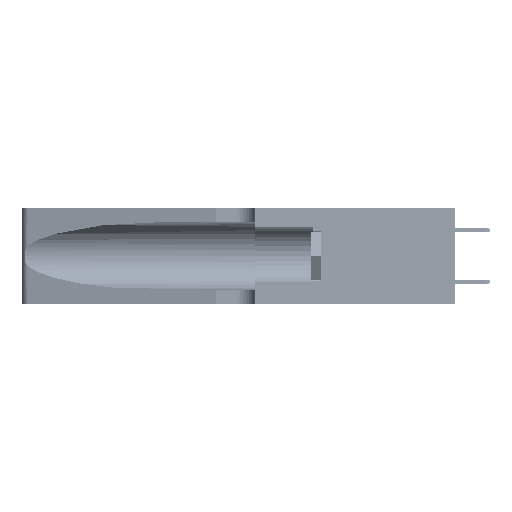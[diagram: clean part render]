
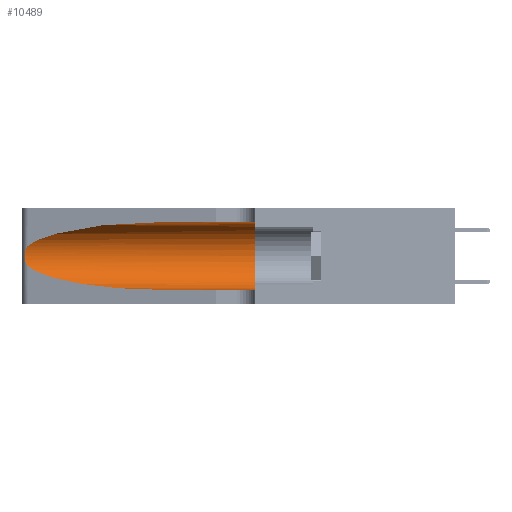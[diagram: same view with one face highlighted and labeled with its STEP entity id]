
A CAD part, left-side view. The second image highlights one B-rep face of the part: STEP entity #10489.
In plain terms, the highlighted cylindrical face has radius 3.308 mm (diameter 6.617 mm), a partial arc.
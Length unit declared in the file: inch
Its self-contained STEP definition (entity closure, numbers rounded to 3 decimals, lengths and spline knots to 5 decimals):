
#362 = ORIENTED_EDGE ( 'NONE', *, *, #37674, .F. ) ;
#454 = AXIS2_PLACEMENT_3D ( 'NONE', #43914, #44186, #11364 ) ;
#1135 = CARTESIAN_POINT ( 'NONE',  ( 0.1305, 1.61858, 0.05475 ) ) ;
#1635 = ORIENTED_EDGE ( 'NONE', *, *, #9774, .T. ) ;
#2029 = EDGE_CURVE ( 'NONE', #44877, #31511, #16882, .T. ) ;
#2065 = CARTESIAN_POINT ( 'NONE',  ( 0.1305, 0.35, 0.05475 ) ) ;
#3035 = DIRECTION ( 'NONE',  ( 0., -1., 0. ) ) ;
#4154 = CARTESIAN_POINT ( 'NONE',  ( 0.25555, 1.22994, 0.2215 ) ) ;
#4915 = VERTEX_POINT ( 'NONE', #21730 ) ;
#5447 =( BOUNDED_CURVE ( )  B_SPLINE_CURVE ( 3, ( #11576, #44661, #23521, #12105 ),
 .UNSPECIFIED., .F., .F. ) 
 B_SPLINE_CURVE_WITH_KNOTS ( ( 4, 4 ),
 ( 3.44316, 4.71239 ),
 .UNSPECIFIED. ) 
 CURVE ( )  GEOMETRIC_REPRESENTATION_ITEM ( )  RATIONAL_B_SPLINE_CURVE ( ( 1., 0.87, 0.87, 1. ) ) 
 REPRESENTATION_ITEM ( '' )  );
#7596 = CARTESIAN_POINT ( 'NONE',  ( 0.1305, 0.35, 0.31525 ) ) ;
#9774 = EDGE_CURVE ( 'NONE', #36606, #4915, #38628, .T. ) ;
#10489 = ADVANCED_FACE ( 'NONE', ( #14635 ), #14356, .F. ) ;
#10690 = CARTESIAN_POINT ( 'NONE',  ( 0.25487, 1.22718, 0.22369 ) ) ;
#10956 = CARTESIAN_POINT ( 'NONE',  ( 0.1305, 0.72297, 0.31525 ) ) ;
#11364 = DIRECTION ( 'NONE',  ( 0., 0., -1. ) ) ;
#11576 = CARTESIAN_POINT ( 'NONE',  ( 0.25487, 1.22718, 0.14631 ) ) ;
#11835 = ORIENTED_EDGE ( 'NONE', *, *, #2029, .T. ) ;
#12105 = CARTESIAN_POINT ( 'NONE',  ( 0.1305, 0.72297, 0.05475 ) ) ;
#12561 = CARTESIAN_POINT ( 'NONE',  ( 0.25487, 1.22718, 0.22369 ) ) ;
#12828 = CARTESIAN_POINT ( 'NONE',  ( 0.26075, 1.23896, 0.178 ) ) ;
#13082 = CARTESIAN_POINT ( 'NONE',  ( 0.26017, 1.23833, 0.17102 ) ) ;
#13103 = EDGE_CURVE ( 'NONE', #33153, #36606, #24790, .T. ) ;
#14356 = CYLINDRICAL_SURFACE ( 'NONE', #454, 0.13025 ) ;
#14635 = FACE_OUTER_BOUND ( 'NONE', #35063, .T. ) ;
#14978 = LINE ( 'NONE', #30992, #28762 ) ;
#14979 = VECTOR ( 'NONE', #42076, 39.37008 ) ;
#16092 = CARTESIAN_POINT ( 'NONE',  ( 0.25639, 1.23186, 0.15144 ) ) ;
#16882 = LINE ( 'NONE', #1135, #14979 ) ;
#16906 = CARTESIAN_POINT ( 'NONE',  ( 0.25789, 1.23486, 0.15765 ) ) ;
#18568 = CARTESIAN_POINT ( 'NONE',  ( 0.1305, 0.35, 0.185 ) ) ;
#21239 = CARTESIAN_POINT ( 'NONE',  ( 0.25854, 1.2359, 0.20912 ) ) ;
#21365 = AXIS2_PLACEMENT_3D ( 'NONE', #18568, #46761, #50561 ) ;
#21730 = CARTESIAN_POINT ( 'NONE',  ( 0.25487, 1.22718, 0.14631 ) ) ;
#23521 = CARTESIAN_POINT ( 'NONE',  ( 0.18966, 0.96281, 0.05475 ) ) ;
#23794 = VERTEX_POINT ( 'NONE', #7596 ) ;
#24790 =( BOUNDED_CURVE ( )  B_SPLINE_CURVE ( 3, ( #10956, #48110, #35371, #10690 ),
 .UNSPECIFIED., .F., .F. ) 
 B_SPLINE_CURVE_WITH_KNOTS ( ( 4, 4 ),
 ( 1.5708, 2.84003 ),
 .UNSPECIFIED. ) 
 CURVE ( )  GEOMETRIC_REPRESENTATION_ITEM ( )  RATIONAL_B_SPLINE_CURVE ( ( 1., 0.87, 0.87, 1. ) ) 
 REPRESENTATION_ITEM ( '' )  );
#25047 = CARTESIAN_POINT ( 'NONE',  ( 0.25787, 1.23484, 0.2124 ) ) ;
#25507 = CARTESIAN_POINT ( 'NONE',  ( 0.25487, 1.22718, 0.22369 ) ) ;
#28430 = CARTESIAN_POINT ( 'NONE',  ( 0.1305, 0.72297, 0.31525 ) ) ;
#28762 = VECTOR ( 'NONE', #3035, 39.37008 ) ;
#28849 = ORIENTED_EDGE ( 'NONE', *, *, #13103, .T. ) ;
#30511 = CARTESIAN_POINT ( 'NONE',  ( 0.1305, 0.72297, 0.05475 ) ) ;
#30885 = CIRCLE ( 'NONE', #21365, 0.13025 ) ;
#30992 = CARTESIAN_POINT ( 'NONE',  ( 0.1305, 1.61858, 0.31525 ) ) ;
#31511 = VERTEX_POINT ( 'NONE', #2065 ) ;
#33153 = VERTEX_POINT ( 'NONE', #28430 ) ;
#33811 = ORIENTED_EDGE ( 'NONE', *, *, #49538, .T. ) ;
#35063 = EDGE_LOOP ( 'NONE', ( #28849, #1635, #33811, #11835, #39502, #362 ) ) ;
#35371 = CARTESIAN_POINT ( 'NONE',  ( 0.2373, 1.15595, 0.28018 ) ) ;
#36606 = VERTEX_POINT ( 'NONE', #25507 ) ;
#36716 = CARTESIAN_POINT ( 'NONE',  ( 0.25639, 1.23184, 0.21858 ) ) ;
#37674 = EDGE_CURVE ( 'NONE', #33153, #23794, #14978, .T. ) ;
#38628 = B_SPLINE_CURVE_WITH_KNOTS ( 'NONE', 3,
 ( #12561, #4154, #36716, #25047, #21239, #53257, #45643, #12828, #13082, #49442, #16906, #16092, #44845, #53523 ),
 .UNSPECIFIED., .F., .F.,
 ( 4, 2, 2, 2, 2, 2, 4 ),
 ( 0., 0.00027, 0.00053, 0.00107, 0.0016, 0.00187, 0.00214 ),
 .UNSPECIFIED. ) ;
#39502 = ORIENTED_EDGE ( 'NONE', *, *, #43336, .F. ) ;
#42076 = DIRECTION ( 'NONE',  ( 0., -1., 0. ) ) ;
#43336 = EDGE_CURVE ( 'NONE', #23794, #31511, #30885, .T. ) ;
#43914 = CARTESIAN_POINT ( 'NONE',  ( 0.1305, 1.61858, 0.185 ) ) ;
#44186 = DIRECTION ( 'NONE',  ( 0., -1., 0. ) ) ;
#44661 = CARTESIAN_POINT ( 'NONE',  ( 0.2373, 1.15595, 0.08982 ) ) ;
#44845 = CARTESIAN_POINT ( 'NONE',  ( 0.25555, 1.22993, 0.14849 ) ) ;
#44877 = VERTEX_POINT ( 'NONE', #30511 ) ;
#45643 = CARTESIAN_POINT ( 'NONE',  ( 0.26075, 1.23896, 0.19203 ) ) ;
#46761 = DIRECTION ( 'NONE',  ( 0., 1., 0. ) ) ;
#48110 = CARTESIAN_POINT ( 'NONE',  ( 0.18966, 0.96281, 0.31525 ) ) ;
#49442 = CARTESIAN_POINT ( 'NONE',  ( 0.25856, 1.23593, 0.16098 ) ) ;
#49538 = EDGE_CURVE ( 'NONE', #4915, #44877, #5447, .T. ) ;
#50561 = DIRECTION ( 'NONE',  ( 0., 0., 1. ) ) ;
#53257 = CARTESIAN_POINT ( 'NONE',  ( 0.26018, 1.23835, 0.19895 ) ) ;
#53523 = CARTESIAN_POINT ( 'NONE',  ( 0.25487, 1.22718, 0.14631 ) ) ;
